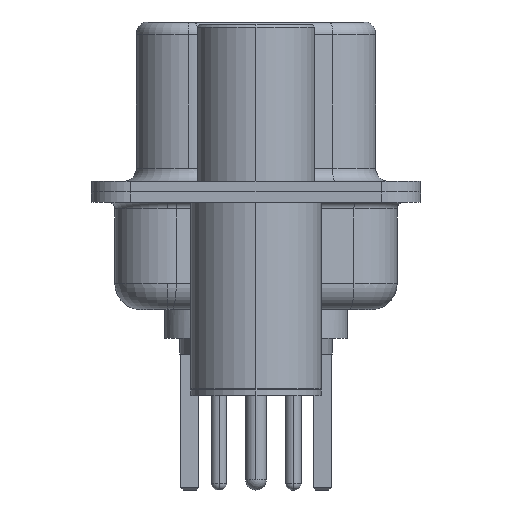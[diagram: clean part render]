
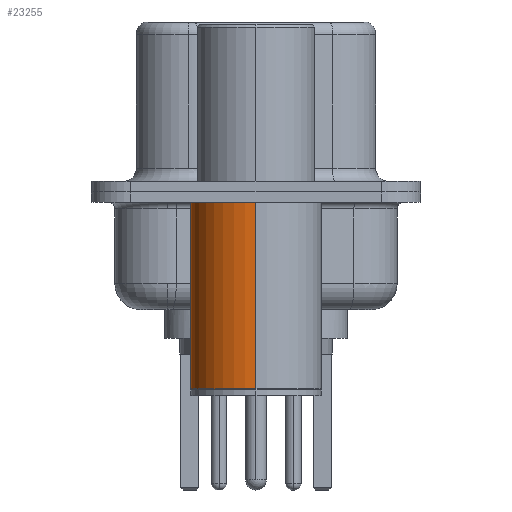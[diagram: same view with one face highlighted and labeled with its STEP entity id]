
A CAD part, left-side view. The second image highlights one B-rep face of the part: STEP entity #23255.
In plain terms, the highlighted cylindrical face has radius 2.5 mm (diameter 5 mm), a partial arc.
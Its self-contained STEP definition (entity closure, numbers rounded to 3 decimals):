
#3506 = EDGE_CURVE ( 'NONE', #12153, #25654, #19625, .T. ) ;
#4822 = DIRECTION ( 'NONE',  ( 0., 0., 1. ) ) ;
#5704 = CARTESIAN_POINT ( 'NONE',  ( 0., 0., 0.581 ) ) ;
#6054 = EDGE_CURVE ( 'NONE', #12153, #27577, #20932, .T. ) ;
#6360 = ORIENTED_EDGE ( 'NONE', *, *, #27104, .F. ) ;
#6516 = CARTESIAN_POINT ( 'NONE',  ( -2.5, 0., 0.581 ) ) ;
#8068 = DIRECTION ( 'NONE',  ( 1., 0., 0. ) ) ;
#8158 = DIRECTION ( 'NONE',  ( 0., 0., 1. ) ) ;
#8898 = CARTESIAN_POINT ( 'NONE',  ( -2.5, 0., -0.4 ) ) ;
#9723 = AXIS2_PLACEMENT_3D ( 'NONE', #5704, #8158, #8068 ) ;
#9748 = VERTEX_POINT ( 'NONE', #8898 ) ;
#10686 = EDGE_CURVE ( 'NONE', #25654, #9748, #28641, .T. ) ;
#10942 = DIRECTION ( 'NONE',  ( 0., 0., 1. ) ) ;
#12153 = VERTEX_POINT ( 'NONE', #14338 ) ;
#12270 = DIRECTION ( 'NONE',  ( 0., 0., 1. ) ) ;
#13043 = CARTESIAN_POINT ( 'NONE',  ( 2.5, 0., 0.581 ) ) ;
#13362 = ORIENTED_EDGE ( 'NONE', *, *, #6054, .F. ) ;
#13547 = CARTESIAN_POINT ( 'NONE',  ( -2.5, 0., -7.525 ) ) ;
#14338 = CARTESIAN_POINT ( 'NONE',  ( 2.5, 0., -7.525 ) ) ;
#14552 = FACE_OUTER_BOUND ( 'NONE', #23549, .T. ) ;
#14922 = DIRECTION ( 'NONE',  ( 1., 0., 0. ) ) ;
#15236 = CYLINDRICAL_SURFACE ( 'NONE', #9723, 2.5 ) ;
#15303 = ORIENTED_EDGE ( 'NONE', *, *, #10686, .T. ) ;
#15482 = AXIS2_PLACEMENT_3D ( 'NONE', #19096, #12270, #14922 ) ;
#17173 = ORIENTED_EDGE ( 'NONE', *, *, #3506, .T. ) ;
#17631 = DIRECTION ( 'NONE',  ( 0., 0., 1. ) ) ;
#19096 = CARTESIAN_POINT ( 'NONE',  ( 0., 0., -7.525 ) ) ;
#19625 = CIRCLE ( 'NONE', #15482, 2.5 ) ;
#20932 = LINE ( 'NONE', #13043, #21297 ) ;
#21297 = VECTOR ( 'NONE', #17631, 1000. ) ;
#21949 = CIRCLE ( 'NONE', #28419, 2.5 ) ;
#22673 = VECTOR ( 'NONE', #10942, 1000. ) ;
#22781 = DIRECTION ( 'NONE',  ( 1., 0., 0. ) ) ;
#23255 = ADVANCED_FACE ( 'NONE', ( #14552 ), #15236, .T. ) ;
#23549 = EDGE_LOOP ( 'NONE', ( #17173, #15303, #6360, #13362 ) ) ;
#24762 = CARTESIAN_POINT ( 'NONE',  ( 0., 0., -0.4 ) ) ;
#25654 = VERTEX_POINT ( 'NONE', #13547 ) ;
#26585 = CARTESIAN_POINT ( 'NONE',  ( 2.5, 0., -0.4 ) ) ;
#27104 = EDGE_CURVE ( 'NONE', #27577, #9748, #21949, .T. ) ;
#27577 = VERTEX_POINT ( 'NONE', #26585 ) ;
#28419 = AXIS2_PLACEMENT_3D ( 'NONE', #24762, #4822, #22781 ) ;
#28641 = LINE ( 'NONE', #6516, #22673 ) ;
